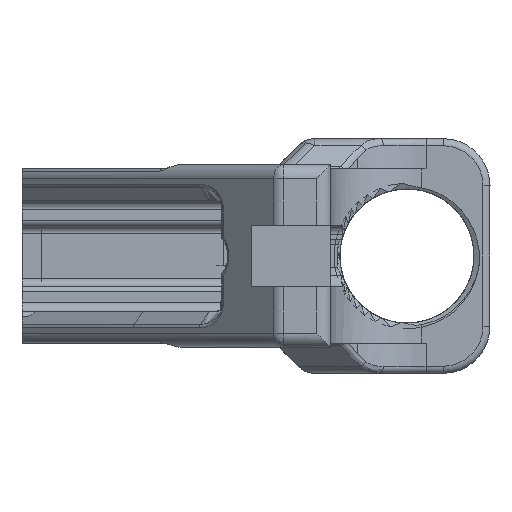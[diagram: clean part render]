
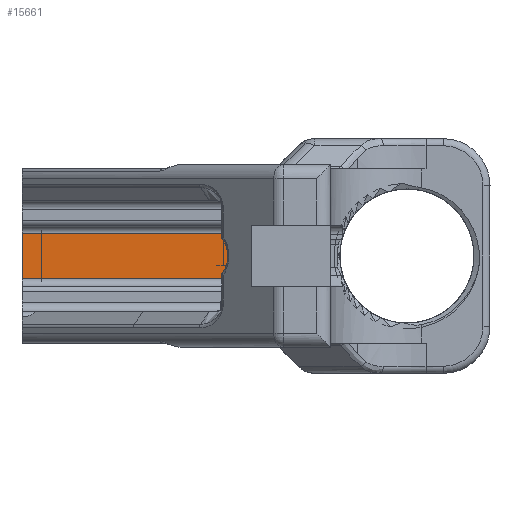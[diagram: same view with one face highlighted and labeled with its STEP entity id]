
A CAD part, left-side view. The second image highlights one B-rep face of the part: STEP entity #15661.
In plain terms, the highlighted planar face has unit normal (-1, 0, 0).
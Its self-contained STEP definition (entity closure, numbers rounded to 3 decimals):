
#946 = CARTESIAN_POINT ( 'NONE',  ( -40.772, 44.245, 46.89 ) ) ;
#1111 = CARTESIAN_POINT ( 'NONE',  ( -40.772, 66.175, 46.89 ) ) ;
#1448 = CARTESIAN_POINT ( 'NONE',  ( -40.772, 66.175, 54.779 ) ) ;
#2213 = ORIENTED_EDGE ( 'NONE', *, *, #19342, .F. ) ;
#2338 = EDGE_CURVE ( 'NONE', #38000, #32155, #30872, .T. ) ;
#4776 = CARTESIAN_POINT ( 'NONE',  ( -40.772, 22.315, 46.89 ) ) ;
#5258 = DIRECTION ( 'NONE',  ( 0., 1., 0. ) ) ;
#6838 = LINE ( 'NONE', #1448, #14532 ) ;
#6934 = LINE ( 'NONE', #27734, #17031 ) ;
#7513 = VECTOR ( 'NONE', #34157, 1000. ) ;
#9396 = DIRECTION ( 'NONE',  ( 1., 0., 0. ) ) ;
#9517 = ORIENTED_EDGE ( 'NONE', *, *, #13764, .F. ) ;
#11539 = CARTESIAN_POINT ( 'NONE',  ( -40.772, 0.385, 23.467 ) ) ;
#12911 = CARTESIAN_POINT ( 'NONE',  ( -40.772, 0.385, 46.89 ) ) ;
#13764 = EDGE_CURVE ( 'NONE', #20996, #38596, #6934, .T. ) ;
#14532 = VECTOR ( 'NONE', #20646, 1000. ) ;
#15661 = ADVANCED_FACE ( 'NONE', ( #41010 ), #39439, .F. ) ;
#17031 = VECTOR ( 'NONE', #5258, 1000. ) ;
#17593 = EDGE_LOOP ( 'NONE', ( #21795, #2213, #9517, #48514 ) ) ;
#18844 = EDGE_CURVE ( 'NONE', #20996, #38000, #36449, .T. ) ;
#19342 = EDGE_CURVE ( 'NONE', #38596, #32155, #6838, .T. ) ;
#19418 = CARTESIAN_POINT ( 'NONE',  ( -40.772, 0.385, 37.237 ) ) ;
#20646 = DIRECTION ( 'NONE',  ( 0., 0., 1. ) ) ;
#20996 = VERTEX_POINT ( 'NONE', #19418 ) ;
#21795 = ORIENTED_EDGE ( 'NONE', *, *, #2338, .T. ) ;
#23776 = CARTESIAN_POINT ( 'NONE',  ( -40.772, 0.385, 46.89 ) ) ;
#26389 = CARTESIAN_POINT ( 'NONE',  ( -40.772, 66.175, 46.89 ) ) ;
#27734 = CARTESIAN_POINT ( 'NONE',  ( -40.772, 66.175, 37.237 ) ) ;
#30872 = B_SPLINE_CURVE_WITH_KNOTS ( 'NONE', 3,
 ( #23776, #4776, #946, #1111 ),
 .UNSPECIFIED., .F., .F.,
 ( 4, 4 ),
 ( 0., 1. ),
 .UNSPECIFIED. ) ;
#31583 = CARTESIAN_POINT ( 'NONE',  ( -40.772, 66.175, 37.237 ) ) ;
#32011 = CARTESIAN_POINT ( 'NONE',  ( -40.772, 66.175, 42.064 ) ) ;
#32155 = VERTEX_POINT ( 'NONE', #26389 ) ;
#33977 = AXIS2_PLACEMENT_3D ( 'NONE', #32011, #9396, #35811 ) ;
#34157 = DIRECTION ( 'NONE',  ( 0., 0., 1. ) ) ;
#35811 = DIRECTION ( 'NONE',  ( 0., 1., 0. ) ) ;
#36449 = LINE ( 'NONE', #11539, #7513 ) ;
#38000 = VERTEX_POINT ( 'NONE', #12911 ) ;
#38596 = VERTEX_POINT ( 'NONE', #31583 ) ;
#39439 = PLANE ( 'NONE',  #33977 ) ;
#41010 = FACE_OUTER_BOUND ( 'NONE', #17593, .T. ) ;
#48514 = ORIENTED_EDGE ( 'NONE', *, *, #18844, .T. ) ;
